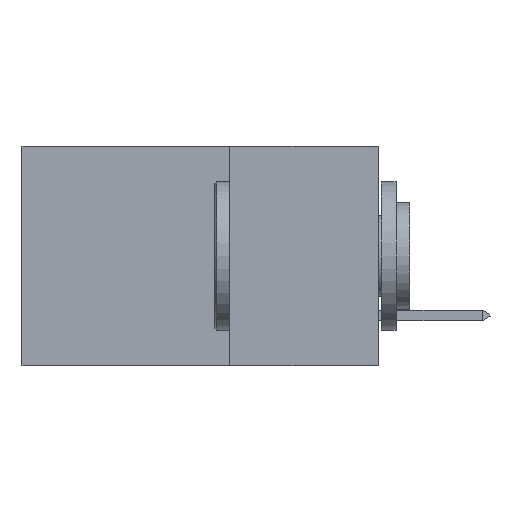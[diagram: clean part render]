
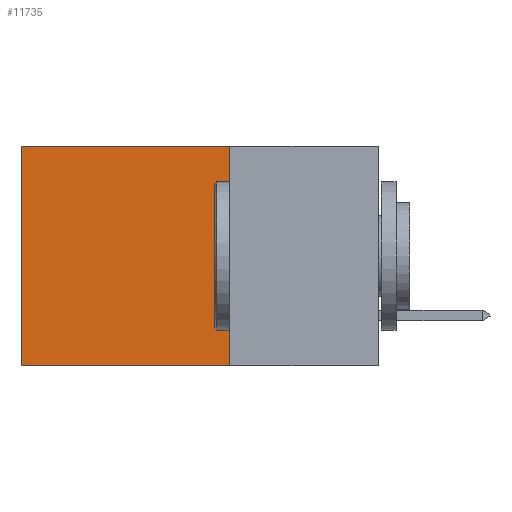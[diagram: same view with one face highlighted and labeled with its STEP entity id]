
A CAD part, left-side view. The second image highlights one B-rep face of the part: STEP entity #11735.
In plain terms, the highlighted planar face has unit normal (-1, 0, 0).
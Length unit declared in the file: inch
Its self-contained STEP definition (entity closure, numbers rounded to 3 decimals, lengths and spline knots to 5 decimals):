
#231 = AXIS2_PLACEMENT_3D ( 'NONE', #4409, #7482, #12368 ) ;
#507 = DIRECTION ( 'NONE',  ( 0., 0., -1. ) ) ;
#640 = ORIENTED_EDGE ( 'NONE', *, *, #8264, .T. ) ;
#842 = VECTOR ( 'NONE', #11241, 39.37008 ) ;
#2241 = CARTESIAN_POINT ( 'NONE',  ( 0.298, 0.25, 0. ) ) ;
#2779 = EDGE_CURVE ( 'NONE', #5243, #10719, #8987, .T. ) ;
#2846 = ORIENTED_EDGE ( 'NONE', *, *, #8876, .T. ) ;
#3316 = EDGE_LOOP ( 'NONE', ( #2846, #5298, #6670, #640 ) ) ;
#3594 = DIRECTION ( 'NONE',  ( 0., 1., 0. ) ) ;
#4409 = CARTESIAN_POINT ( 'NONE',  ( 0.298, 0.25, 0. ) ) ;
#4474 = CARTESIAN_POINT ( 'NONE',  ( 0.298, 0.25, -0.37 ) ) ;
#4883 = VECTOR ( 'NONE', #507, 39.37008 ) ;
#5243 = VERTEX_POINT ( 'NONE', #6013 ) ;
#5298 = ORIENTED_EDGE ( 'NONE', *, *, #7502, .F. ) ;
#5433 = CARTESIAN_POINT ( 'NONE',  ( 0.298, 0.6, 0. ) ) ;
#5837 = VECTOR ( 'NONE', #3594, 39.37008 ) ;
#6013 = CARTESIAN_POINT ( 'NONE',  ( 0.298, 0.25, 0. ) ) ;
#6336 = DIRECTION ( 'NONE',  ( 0., 1., 0. ) ) ;
#6470 = VECTOR ( 'NONE', #6336, 39.37008 ) ;
#6670 = ORIENTED_EDGE ( 'NONE', *, *, #2779, .F. ) ;
#7481 = CARTESIAN_POINT ( 'NONE',  ( 0.298, 0.25, 0. ) ) ;
#7482 = DIRECTION ( 'NONE',  ( 1., 0., 0. ) ) ;
#7502 = EDGE_CURVE ( 'NONE', #10719, #7507, #9120, .T. ) ;
#7507 = VERTEX_POINT ( 'NONE', #7607 ) ;
#7546 = LINE ( 'NONE', #5433, #4883 ) ;
#7607 = CARTESIAN_POINT ( 'NONE',  ( 0.298, 0.6, -0.37 ) ) ;
#8264 = EDGE_CURVE ( 'NONE', #5243, #11036, #8654, .T. ) ;
#8654 = LINE ( 'NONE', #7481, #5837 ) ;
#8876 = EDGE_CURVE ( 'NONE', #11036, #7507, #7546, .T. ) ;
#8987 = LINE ( 'NONE', #2241, #842 ) ;
#9120 = LINE ( 'NONE', #11347, #6470 ) ;
#9453 = PLANE ( 'NONE',  #231 ) ;
#10719 = VERTEX_POINT ( 'NONE', #4474 ) ;
#10999 = FACE_OUTER_BOUND ( 'NONE', #3316, .T. ) ;
#11036 = VERTEX_POINT ( 'NONE', #12172 ) ;
#11241 = DIRECTION ( 'NONE',  ( 0., 0., -1. ) ) ;
#11347 = CARTESIAN_POINT ( 'NONE',  ( 0.298, 0.25, -0.37 ) ) ;
#11735 = ADVANCED_FACE ( 'NONE', ( #10999 ), #9453, .F. ) ;
#12172 = CARTESIAN_POINT ( 'NONE',  ( 0.298, 0.6, 0. ) ) ;
#12368 = DIRECTION ( 'NONE',  ( 0., 0., -1. ) ) ;
